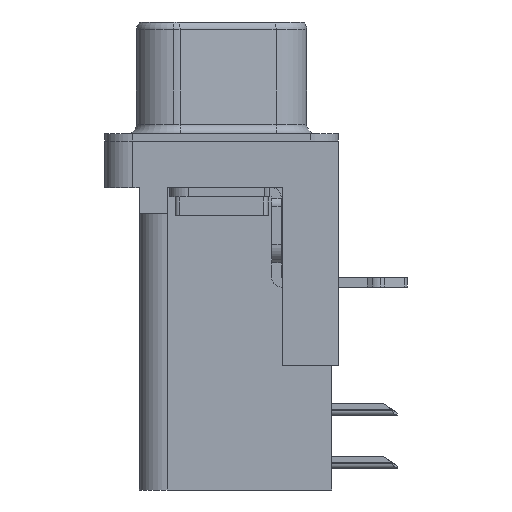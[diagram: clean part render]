
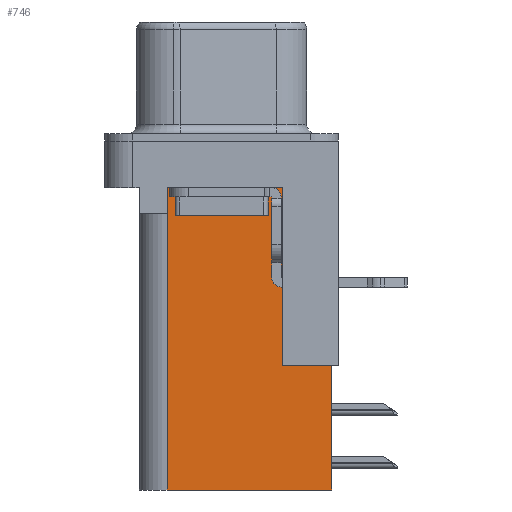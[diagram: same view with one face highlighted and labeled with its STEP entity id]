
A CAD part, left-side view. The second image highlights one B-rep face of the part: STEP entity #746.
In plain terms, the highlighted planar face has unit normal (-1, 0, 0).
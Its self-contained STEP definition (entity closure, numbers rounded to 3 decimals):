
#89 = VERTEX_POINT ( 'NONE', #11226 ) ;
#173 = ORIENTED_EDGE ( 'NONE', *, *, #14080, .F. ) ;
#314 = DIRECTION ( 'NONE',  ( 0., 1., 0. ) ) ;
#746 = ADVANCED_FACE ( 'NONE', ( #13507 ), #14605, .F. ) ;
#918 = VERTEX_POINT ( 'NONE', #24990 ) ;
#1036 = ORIENTED_EDGE ( 'NONE', *, *, #13760, .F. ) ;
#1557 = VERTEX_POINT ( 'NONE', #9172 ) ;
#1804 = VECTOR ( 'NONE', #3178, 1000. ) ;
#2103 = LINE ( 'NONE', #10464, #17659 ) ;
#2257 = CARTESIAN_POINT ( 'NONE',  ( 3.79, -5.925, -12.05 ) ) ;
#2899 = ORIENTED_EDGE ( 'NONE', *, *, #5438, .T. ) ;
#3178 = DIRECTION ( 'NONE',  ( 0., 1., 0. ) ) ;
#3588 = VECTOR ( 'NONE', #8084, 1000. ) ;
#3812 = CARTESIAN_POINT ( 'NONE',  ( 3.79, -5.925, -18.76 ) ) ;
#4015 = VERTEX_POINT ( 'NONE', #20580 ) ;
#4105 = LINE ( 'NONE', #23653, #24281 ) ;
#4885 = VECTOR ( 'NONE', #8366, 1000. ) ;
#5438 = EDGE_CURVE ( 'NONE', #18016, #89, #4105, .T. ) ;
#5658 = CARTESIAN_POINT ( 'NONE',  ( 3.79, -5.925, -2. ) ) ;
#5986 = VECTOR ( 'NONE', #14016, 1000. ) ;
#6362 = LINE ( 'NONE', #16814, #1804 ) ;
#6827 = EDGE_LOOP ( 'NONE', ( #17794, #13982, #17610, #173, #10051, #1036, #2899, #20396 ) ) ;
#7486 = VECTOR ( 'NONE', #20266, 1000. ) ;
#7580 = VECTOR ( 'NONE', #23264, 1000. ) ;
#8084 = DIRECTION ( 'NONE',  ( 0., 0., 1. ) ) ;
#8109 = LINE ( 'NONE', #8517, #7486 ) ;
#8366 = DIRECTION ( 'NONE',  ( 0., 0., -1. ) ) ;
#8517 = CARTESIAN_POINT ( 'NONE',  ( 3.79, 0., -3.9 ) ) ;
#8742 = LINE ( 'NONE', #19806, #3588 ) ;
#9172 = CARTESIAN_POINT ( 'NONE',  ( 3.79, 2.895, -2.5 ) ) ;
#9800 = EDGE_CURVE ( 'NONE', #17267, #4015, #16348, .T. ) ;
#9942 = EDGE_CURVE ( 'NONE', #918, #19121, #8109, .T. ) ;
#10051 = ORIENTED_EDGE ( 'NONE', *, *, #9800, .F. ) ;
#10243 = CARTESIAN_POINT ( 'NONE',  ( 3.79, -3.295, -18.76 ) ) ;
#10464 = CARTESIAN_POINT ( 'NONE',  ( 3.79, 2.925, -18.76 ) ) ;
#11226 = CARTESIAN_POINT ( 'NONE',  ( 3.79, -3.295, -12.05 ) ) ;
#12003 = CARTESIAN_POINT ( 'NONE',  ( 3.79, -3.295, -18.76 ) ) ;
#13507 = FACE_OUTER_BOUND ( 'NONE', #6827, .T. ) ;
#13760 = EDGE_CURVE ( 'NONE', #18016, #17267, #14020, .T. ) ;
#13982 = ORIENTED_EDGE ( 'NONE', *, *, #24536, .T. ) ;
#14016 = DIRECTION ( 'NONE',  ( 0., 1., 0. ) ) ;
#14020 = LINE ( 'NONE', #5658, #7580 ) ;
#14080 = EDGE_CURVE ( 'NONE', #4015, #19121, #2103, .T. ) ;
#14180 = AXIS2_PLACEMENT_3D ( 'NONE', #10243, #15230, #314 ) ;
#14605 = PLANE ( 'NONE',  #14180 ) ;
#15230 = DIRECTION ( 'NONE',  ( 1., 0., 0. ) ) ;
#16348 = LINE ( 'NONE', #12003, #5986 ) ;
#16814 = CARTESIAN_POINT ( 'NONE',  ( 3.79, -3.295, -2.5 ) ) ;
#17267 = VERTEX_POINT ( 'NONE', #3812 ) ;
#17610 = ORIENTED_EDGE ( 'NONE', *, *, #9942, .T. ) ;
#17659 = VECTOR ( 'NONE', #22252, 1000. ) ;
#17794 = ORIENTED_EDGE ( 'NONE', *, *, #19499, .T. ) ;
#18016 = VERTEX_POINT ( 'NONE', #2257 ) ;
#19121 = VERTEX_POINT ( 'NONE', #23465 ) ;
#19499 = EDGE_CURVE ( 'NONE', #22921, #1557, #6362, .T. ) ;
#19806 = CARTESIAN_POINT ( 'NONE',  ( 3.79, -3.295, -18.76 ) ) ;
#19868 = LINE ( 'NONE', #20111, #4885 ) ;
#20111 = CARTESIAN_POINT ( 'NONE',  ( 3.79, 2.895, -3.9 ) ) ;
#20266 = DIRECTION ( 'NONE',  ( 0., 1., 0. ) ) ;
#20328 = EDGE_CURVE ( 'NONE', #89, #22921, #8742, .T. ) ;
#20396 = ORIENTED_EDGE ( 'NONE', *, *, #20328, .T. ) ;
#20580 = CARTESIAN_POINT ( 'NONE',  ( 3.79, 2.925, -18.76 ) ) ;
#22252 = DIRECTION ( 'NONE',  ( 0., 0., 1. ) ) ;
#22562 = DIRECTION ( 'NONE',  ( 0., 1., 0. ) ) ;
#22844 = CARTESIAN_POINT ( 'NONE',  ( 3.79, -3.295, -2.5 ) ) ;
#22921 = VERTEX_POINT ( 'NONE', #22844 ) ;
#23264 = DIRECTION ( 'NONE',  ( 0., 0., -1. ) ) ;
#23465 = CARTESIAN_POINT ( 'NONE',  ( 3.79, 2.925, -3.9 ) ) ;
#23653 = CARTESIAN_POINT ( 'NONE',  ( 3.79, -6.295, -12.05 ) ) ;
#24281 = VECTOR ( 'NONE', #22562, 1000. ) ;
#24536 = EDGE_CURVE ( 'NONE', #1557, #918, #19868, .T. ) ;
#24990 = CARTESIAN_POINT ( 'NONE',  ( 3.79, 2.895, -3.9 ) ) ;
